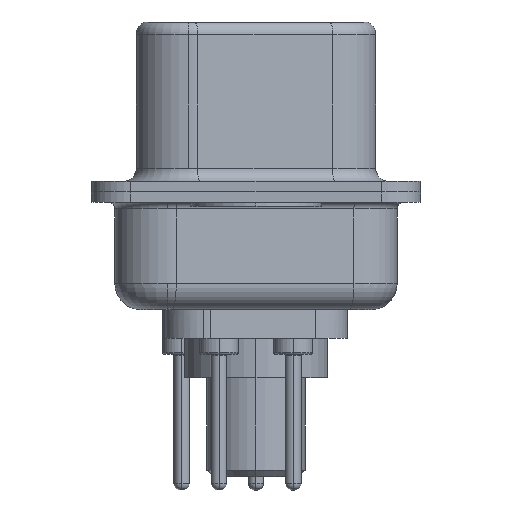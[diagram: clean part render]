
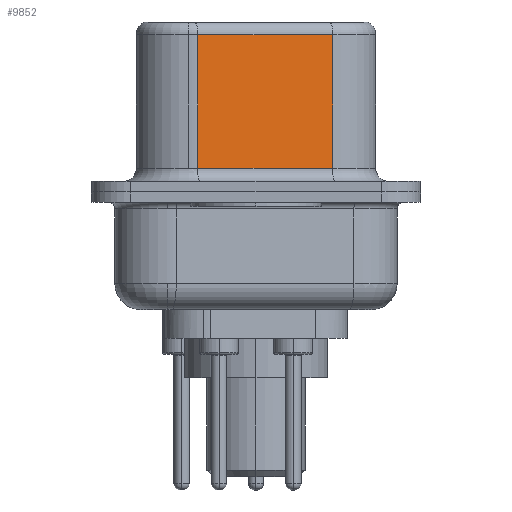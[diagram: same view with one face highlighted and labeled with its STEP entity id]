
A CAD part, left-side view. The second image highlights one B-rep face of the part: STEP entity #9852.
In plain terms, the highlighted planar face has unit normal (-0.985, -0.174, 0).
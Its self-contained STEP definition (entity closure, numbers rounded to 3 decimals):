
#226 = DIRECTION ( 'NONE',  ( 0., 0., -1. ) ) ;
#227 = EDGE_CURVE ( 'NONE', #17703, #15578, #5930, .T. ) ;
#314 = EDGE_LOOP ( 'NONE', ( #998, #16843, #16085, #4016 ) ) ;
#998 = ORIENTED_EDGE ( 'NONE', *, *, #5314, .F. ) ;
#1996 = CARTESIAN_POINT ( 'NONE',  ( 4.585, -2.927, 6.52 ) ) ;
#3185 = LINE ( 'NONE', #13109, #18192 ) ;
#3476 = EDGE_CURVE ( 'NONE', #7400, #17703, #16679, .T. ) ;
#3870 = EDGE_CURVE ( 'NONE', #15578, #11995, #9679, .T. ) ;
#4016 = ORIENTED_EDGE ( 'NONE', *, *, #3870, .T. ) ;
#4338 = CARTESIAN_POINT ( 'NONE',  ( 4.585, -2.927, 0.9 ) ) ;
#5314 = EDGE_CURVE ( 'NONE', #7400, #11995, #3185, .T. ) ;
#5767 = AXIS2_PLACEMENT_3D ( 'NONE', #1996, #15068, #9328 ) ;
#5895 = DIRECTION ( 'NONE',  ( 0., 0., -1. ) ) ;
#5930 = LINE ( 'NONE', #16078, #14509 ) ;
#6470 = FACE_OUTER_BOUND ( 'NONE', #314, .T. ) ;
#6502 = VECTOR ( 'NONE', #15795, 1000. ) ;
#7400 = VERTEX_POINT ( 'NONE', #8414 ) ;
#7600 = PLANE ( 'NONE',  #5767 ) ;
#8414 = CARTESIAN_POINT ( 'NONE',  ( 4.585, -2.927, 6.02 ) ) ;
#8530 = VECTOR ( 'NONE', #14445, 1000. ) ;
#9328 = DIRECTION ( 'NONE',  ( -0.174, 0.985, 0. ) ) ;
#9679 = LINE ( 'NONE', #4338, #8530 ) ;
#9852 = ADVANCED_FACE ( 'NONE', ( #6470 ), #7600, .F. ) ;
#10212 = CARTESIAN_POINT ( 'NONE',  ( 4.585, -2.927, 6.02 ) ) ;
#11995 = VERTEX_POINT ( 'NONE', #14655 ) ;
#12806 = CARTESIAN_POINT ( 'NONE',  ( 3.675, 2.233, 6.02 ) ) ;
#13109 = CARTESIAN_POINT ( 'NONE',  ( 4.585, -2.927, 6.52 ) ) ;
#14445 = DIRECTION ( 'NONE',  ( 0.174, -0.985, 0. ) ) ;
#14509 = VECTOR ( 'NONE', #226, 1000. ) ;
#14655 = CARTESIAN_POINT ( 'NONE',  ( 4.585, -2.927, 0.9 ) ) ;
#15068 = DIRECTION ( 'NONE',  ( 0.985, 0.174, 0. ) ) ;
#15578 = VERTEX_POINT ( 'NONE', #18094 ) ;
#15795 = DIRECTION ( 'NONE',  ( -0.174, 0.985, 0. ) ) ;
#16078 = CARTESIAN_POINT ( 'NONE',  ( 3.675, 2.233, 6.52 ) ) ;
#16085 = ORIENTED_EDGE ( 'NONE', *, *, #227, .T. ) ;
#16679 = LINE ( 'NONE', #10212, #6502 ) ;
#16843 = ORIENTED_EDGE ( 'NONE', *, *, #3476, .T. ) ;
#17703 = VERTEX_POINT ( 'NONE', #12806 ) ;
#18094 = CARTESIAN_POINT ( 'NONE',  ( 3.675, 2.233, 0.9 ) ) ;
#18192 = VECTOR ( 'NONE', #5895, 1000. ) ;
